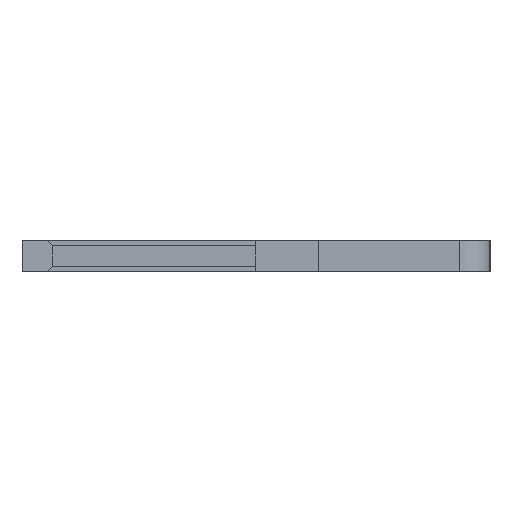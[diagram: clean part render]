
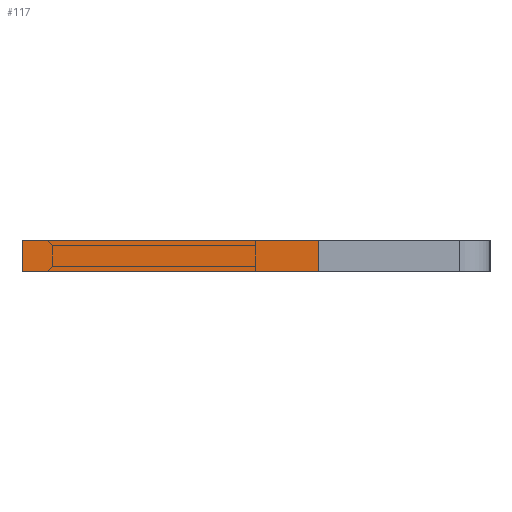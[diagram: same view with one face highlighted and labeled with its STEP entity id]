
A CAD part, left-side view. The second image highlights one B-rep face of the part: STEP entity #117.
In plain terms, the highlighted face is planar.
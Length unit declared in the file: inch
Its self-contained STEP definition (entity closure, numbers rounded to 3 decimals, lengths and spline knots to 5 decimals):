
#4 = VERTEX_POINT ( 'NONE', #1204 ) ;
#52 = EDGE_CURVE ( 'NONE', #4, #672, #1758, .T. ) ;
#100 = LINE ( 'NONE', #549, #1100 ) ;
#117 = ADVANCED_FACE ( 'NONE', ( #2018 ), #515, .F. ) ;
#193 = DIRECTION ( 'NONE',  ( 0., 0., 1. ) ) ;
#275 = EDGE_CURVE ( 'NONE', #2039, #672, #100, .T. ) ;
#289 = CARTESIAN_POINT ( 'NONE',  ( 0.01, 0.15, -0.04 ) ) ;
#314 = DIRECTION ( 'NONE',  ( 0., 1., 0. ) ) ;
#350 = VECTOR ( 'NONE', #314, 39.37008 ) ;
#371 = DIRECTION ( 'NONE',  ( -1., 0., 0. ) ) ;
#394 = AXIS2_PLACEMENT_3D ( 'NONE', #1783, #193, #891 ) ;
#515 = PLANE ( 'NONE',  #394 ) ;
#520 = ORIENTED_EDGE ( 'NONE', *, *, #275, .F. ) ;
#549 = CARTESIAN_POINT ( 'NONE',  ( 0.01, 0.15, -0.04 ) ) ;
#587 = LINE ( 'NONE', #1326, #1369 ) ;
#672 = VERTEX_POINT ( 'NONE', #1106 ) ;
#768 = EDGE_LOOP ( 'NONE', ( #1248, #520, #1653, #854 ) ) ;
#846 = EDGE_CURVE ( 'NONE', #1481, #2039, #1666, .T. ) ;
#854 = ORIENTED_EDGE ( 'NONE', *, *, #972, .T. ) ;
#891 = DIRECTION ( 'NONE',  ( 1., 0., 0. ) ) ;
#938 = DIRECTION ( 'NONE',  ( 0., 1., 0. ) ) ;
#972 = EDGE_CURVE ( 'NONE', #1481, #4, #587, .T. ) ;
#1100 = VECTOR ( 'NONE', #371, 39.37008 ) ;
#1106 = CARTESIAN_POINT ( 'NONE',  ( -0.01, 0.15, -0.04 ) ) ;
#1204 = CARTESIAN_POINT ( 'NONE',  ( -0.01, -0.04, -0.04 ) ) ;
#1248 = ORIENTED_EDGE ( 'NONE', *, *, #52, .T. ) ;
#1312 = DIRECTION ( 'NONE',  ( -1., 0., 0. ) ) ;
#1320 = CARTESIAN_POINT ( 'NONE',  ( 0.01, -0.04, -0.04 ) ) ;
#1326 = CARTESIAN_POINT ( 'NONE',  ( 0.01, -0.04, -0.04 ) ) ;
#1369 = VECTOR ( 'NONE', #1312, 39.37008 ) ;
#1396 = CARTESIAN_POINT ( 'NONE',  ( -0.01, 0.15, -0.04 ) ) ;
#1481 = VERTEX_POINT ( 'NONE', #1320 ) ;
#1653 = ORIENTED_EDGE ( 'NONE', *, *, #846, .F. ) ;
#1666 = LINE ( 'NONE', #2165, #1831 ) ;
#1758 = LINE ( 'NONE', #1396, #350 ) ;
#1783 = CARTESIAN_POINT ( 'NONE',  ( 0.01, 0.15, -0.04 ) ) ;
#1831 = VECTOR ( 'NONE', #938, 39.37008 ) ;
#2018 = FACE_OUTER_BOUND ( 'NONE', #768, .T. ) ;
#2039 = VERTEX_POINT ( 'NONE', #289 ) ;
#2165 = CARTESIAN_POINT ( 'NONE',  ( 0.01, 0.15, -0.04 ) ) ;
